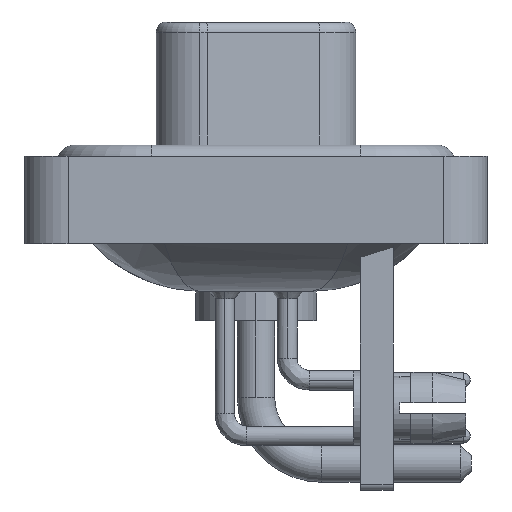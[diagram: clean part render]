
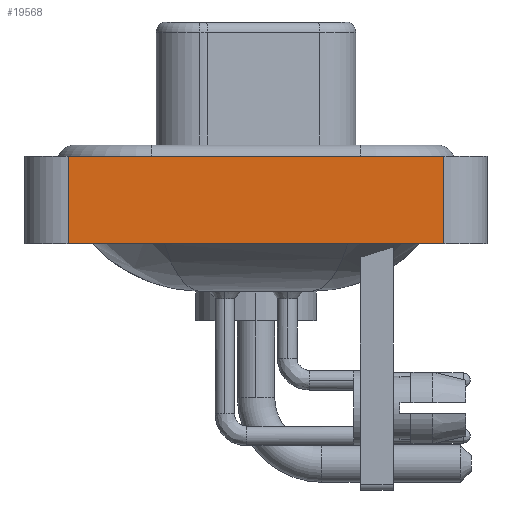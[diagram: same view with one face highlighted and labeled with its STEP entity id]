
A CAD part, left-side view. The second image highlights one B-rep face of the part: STEP entity #19568.
In plain terms, the highlighted planar face has unit normal (-1, 0, 0).
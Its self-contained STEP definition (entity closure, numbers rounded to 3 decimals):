
#187 = CARTESIAN_POINT ( 'NONE',  ( -7.25, -8.55, -3.6 ) ) ;
#367 = ORIENTED_EDGE ( 'NONE', *, *, #7599, .F. ) ;
#462 = CARTESIAN_POINT ( 'NONE',  ( -7.25, -8.55, 0.4 ) ) ;
#4042 = AXIS2_PLACEMENT_3D ( 'NONE', #15984, #10338, #24128 ) ;
#4309 = VECTOR ( 'NONE', #7982, 1000. ) ;
#5028 = CARTESIAN_POINT ( 'NONE',  ( -7.25, -8.55, 0.4 ) ) ;
#5191 = EDGE_CURVE ( 'NONE', #22363, #20138, #9100, .T. ) ;
#5411 = EDGE_CURVE ( 'NONE', #22363, #9014, #6755, .T. ) ;
#5811 = VERTEX_POINT ( 'NONE', #462 ) ;
#6016 = CARTESIAN_POINT ( 'NONE',  ( -7.25, 8.55, -3.6 ) ) ;
#6755 = LINE ( 'NONE', #20683, #10208 ) ;
#7599 = EDGE_CURVE ( 'NONE', #20138, #5811, #11022, .T. ) ;
#7982 = DIRECTION ( 'NONE',  ( 0., 0., 1. ) ) ;
#9014 = VERTEX_POINT ( 'NONE', #20406 ) ;
#9100 = LINE ( 'NONE', #16908, #24848 ) ;
#10208 = VECTOR ( 'NONE', #14675, 1000. ) ;
#10338 = DIRECTION ( 'NONE',  ( -1., 0., 0. ) ) ;
#11022 = LINE ( 'NONE', #5028, #17902 ) ;
#12385 = FACE_OUTER_BOUND ( 'NONE', #17741, .T. ) ;
#13628 = EDGE_CURVE ( 'NONE', #9014, #5811, #17707, .T. ) ;
#13761 = ORIENTED_EDGE ( 'NONE', *, *, #13628, .T. ) ;
#14675 = DIRECTION ( 'NONE',  ( 0., -1., 0. ) ) ;
#14980 = DIRECTION ( 'NONE',  ( 0., 0., 1. ) ) ;
#15984 = CARTESIAN_POINT ( 'NONE',  ( -7.25, -8.55, -3.6 ) ) ;
#16908 = CARTESIAN_POINT ( 'NONE',  ( -7.25, 8.55, -3.6 ) ) ;
#17581 = ORIENTED_EDGE ( 'NONE', *, *, #5191, .F. ) ;
#17707 = LINE ( 'NONE', #187, #4309 ) ;
#17741 = EDGE_LOOP ( 'NONE', ( #13761, #367, #17581, #24843 ) ) ;
#17868 = CARTESIAN_POINT ( 'NONE',  ( -7.25, 8.55, 0.4 ) ) ;
#17902 = VECTOR ( 'NONE', #20242, 1000. ) ;
#19568 = ADVANCED_FACE ( 'NONE', ( #12385 ), #21975, .T. ) ;
#20138 = VERTEX_POINT ( 'NONE', #17868 ) ;
#20242 = DIRECTION ( 'NONE',  ( 0., -1., 0. ) ) ;
#20406 = CARTESIAN_POINT ( 'NONE',  ( -7.25, -8.55, -3.6 ) ) ;
#20683 = CARTESIAN_POINT ( 'NONE',  ( -7.25, -8.55, -3.6 ) ) ;
#21975 = PLANE ( 'NONE',  #4042 ) ;
#22363 = VERTEX_POINT ( 'NONE', #6016 ) ;
#24128 = DIRECTION ( 'NONE',  ( 0., 0., 1. ) ) ;
#24843 = ORIENTED_EDGE ( 'NONE', *, *, #5411, .T. ) ;
#24848 = VECTOR ( 'NONE', #14980, 1000. ) ;
